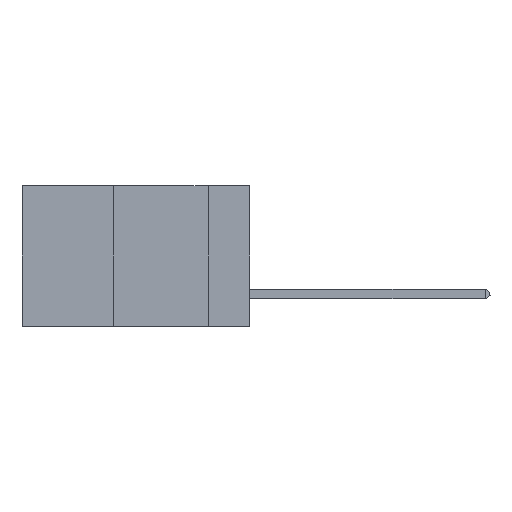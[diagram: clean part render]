
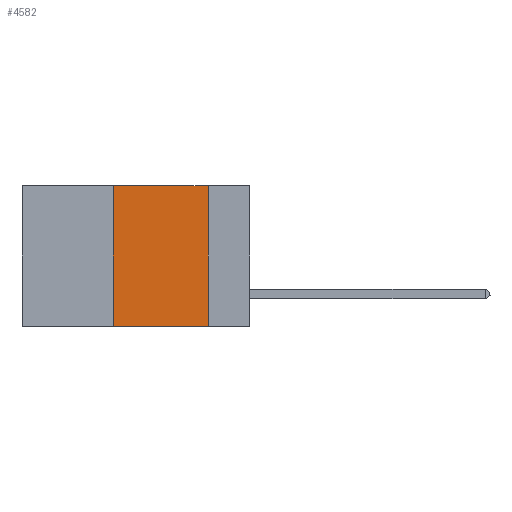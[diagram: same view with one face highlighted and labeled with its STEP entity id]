
A CAD part, left-side view. The second image highlights one B-rep face of the part: STEP entity #4582.
In plain terms, the highlighted planar face has unit normal (-1, 0, 0).
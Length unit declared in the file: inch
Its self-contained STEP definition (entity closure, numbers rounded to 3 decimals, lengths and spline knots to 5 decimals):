
#13 = LINE ( 'NONE', #17412, #4660 ) ;
#470 = CARTESIAN_POINT ( 'NONE',  ( 0., 0.11, 0. ) ) ;
#2454 = EDGE_CURVE ( 'NONE', #22171, #14223, #21694, .T. ) ;
#2850 = PLANE ( 'NONE',  #18949 ) ;
#3000 = DIRECTION ( 'NONE',  ( 1., 0., 0. ) ) ;
#3812 = VECTOR ( 'NONE', #8099, 39.37008 ) ;
#4295 = VECTOR ( 'NONE', #6978, 39.37008 ) ;
#4521 = DIRECTION ( 'NONE',  ( 0., 0., -1. ) ) ;
#4582 = ADVANCED_FACE ( 'NONE', ( #8595 ), #2850, .F. ) ;
#4660 = VECTOR ( 'NONE', #12612, 39.37008 ) ;
#4687 = VERTEX_POINT ( 'NONE', #15938 ) ;
#5846 = CARTESIAN_POINT ( 'NONE',  ( 0., 0.11, 0. ) ) ;
#6978 = DIRECTION ( 'NONE',  ( 0., 0., 1. ) ) ;
#7057 = VERTEX_POINT ( 'NONE', #8358 ) ;
#8099 = DIRECTION ( 'NONE',  ( 0., -1., 0. ) ) ;
#8177 = CARTESIAN_POINT ( 'NONE',  ( 0., 0.6, 0. ) ) ;
#8358 = CARTESIAN_POINT ( 'NONE',  ( 0., 0.36, -0.37 ) ) ;
#8595 = FACE_OUTER_BOUND ( 'NONE', #19806, .T. ) ;
#8896 = CARTESIAN_POINT ( 'NONE',  ( 0., 0.36, 0. ) ) ;
#8923 = EDGE_CURVE ( 'NONE', #7057, #4687, #18946, .T. ) ;
#10681 = CARTESIAN_POINT ( 'NONE',  ( 0., 0.11, -0.37 ) ) ;
#11251 = ORIENTED_EDGE ( 'NONE', *, *, #2454, .F. ) ;
#12612 = DIRECTION ( 'NONE',  ( 0., -1., 0. ) ) ;
#12680 = DIRECTION ( 'NONE',  ( 0., 0., -1. ) ) ;
#14223 = VERTEX_POINT ( 'NONE', #10681 ) ;
#15156 = EDGE_CURVE ( 'NONE', #7057, #14223, #13, .T. ) ;
#15938 = CARTESIAN_POINT ( 'NONE',  ( 0., 0.36, 0. ) ) ;
#16366 = EDGE_CURVE ( 'NONE', #4687, #22171, #21182, .T. ) ;
#17350 = VECTOR ( 'NONE', #12680, 39.37008 ) ;
#17412 = CARTESIAN_POINT ( 'NONE',  ( 0., 0.6, -0.37 ) ) ;
#18533 = CARTESIAN_POINT ( 'NONE',  ( 0., 0.6, 0. ) ) ;
#18940 = ORIENTED_EDGE ( 'NONE', *, *, #15156, .T. ) ;
#18946 = LINE ( 'NONE', #8896, #4295 ) ;
#18949 = AXIS2_PLACEMENT_3D ( 'NONE', #8177, #3000, #4521 ) ;
#19806 = EDGE_LOOP ( 'NONE', ( #11251, #20207, #22375, #18940 ) ) ;
#20207 = ORIENTED_EDGE ( 'NONE', *, *, #16366, .F. ) ;
#21182 = LINE ( 'NONE', #18533, #3812 ) ;
#21694 = LINE ( 'NONE', #470, #17350 ) ;
#22171 = VERTEX_POINT ( 'NONE', #5846 ) ;
#22375 = ORIENTED_EDGE ( 'NONE', *, *, #8923, .F. ) ;
